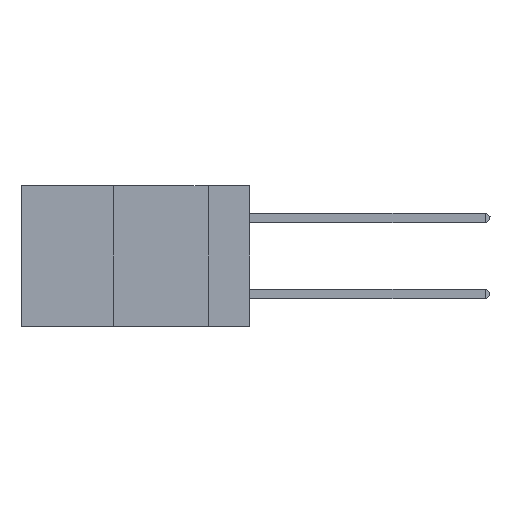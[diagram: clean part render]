
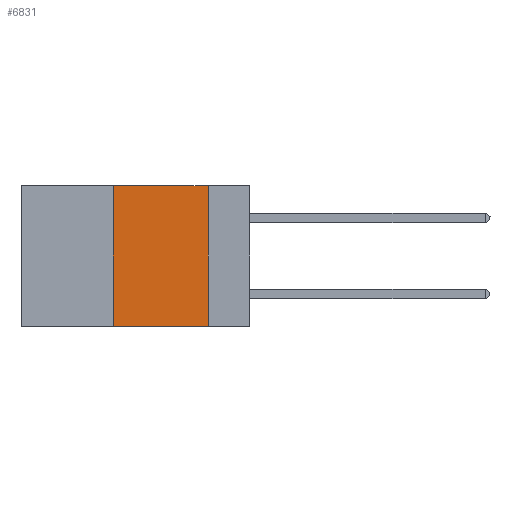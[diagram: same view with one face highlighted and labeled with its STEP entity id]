
A CAD part, left-side view. The second image highlights one B-rep face of the part: STEP entity #6831.
In plain terms, the highlighted planar face has unit normal (-1, 0, 0).
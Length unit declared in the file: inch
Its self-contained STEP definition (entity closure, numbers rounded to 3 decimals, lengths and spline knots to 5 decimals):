
#839 = CARTESIAN_POINT ( 'NONE',  ( 0., 0.6, 0. ) ) ;
#938 = CARTESIAN_POINT ( 'NONE',  ( 0., 0.11, 0. ) ) ;
#1014 = DIRECTION ( 'NONE',  ( 0., 0., -1. ) ) ;
#1046 = DIRECTION ( 'NONE',  ( 0., -1., 0. ) ) ;
#2424 = PLANE ( 'NONE',  #3870 ) ;
#2739 = CARTESIAN_POINT ( 'NONE',  ( 0., 0.11, 0. ) ) ;
#2751 = CARTESIAN_POINT ( 'NONE',  ( 0., 0.36, 0. ) ) ;
#3157 = VECTOR ( 'NONE', #1014, 39.37008 ) ;
#3190 = ORIENTED_EDGE ( 'NONE', *, *, #15618, .F. ) ;
#3303 = VERTEX_POINT ( 'NONE', #2739 ) ;
#3870 = AXIS2_PLACEMENT_3D ( 'NONE', #839, #15048, #6884 ) ;
#4284 = CARTESIAN_POINT ( 'NONE',  ( 0., 0.11, -0.37 ) ) ;
#4734 = EDGE_LOOP ( 'NONE', ( #8311, #4740, #3190, #5533 ) ) ;
#4740 = ORIENTED_EDGE ( 'NONE', *, *, #17905, .F. ) ;
#5424 = LINE ( 'NONE', #5764, #15921 ) ;
#5504 = EDGE_CURVE ( 'NONE', #3303, #11034, #7060, .T. ) ;
#5533 = ORIENTED_EDGE ( 'NONE', *, *, #14988, .T. ) ;
#5764 = CARTESIAN_POINT ( 'NONE',  ( 0., 0.6, -0.37 ) ) ;
#6831 = ADVANCED_FACE ( 'NONE', ( #10636 ), #2424, .F. ) ;
#6884 = DIRECTION ( 'NONE',  ( 0., 0., -1. ) ) ;
#7060 = LINE ( 'NONE', #938, #3157 ) ;
#7329 = LINE ( 'NONE', #12550, #10985 ) ;
#7344 = CARTESIAN_POINT ( 'NONE',  ( 0., 0.36, 0. ) ) ;
#7450 = VERTEX_POINT ( 'NONE', #13889 ) ;
#7642 = LINE ( 'NONE', #2751, #10868 ) ;
#8311 = ORIENTED_EDGE ( 'NONE', *, *, #5504, .F. ) ;
#9996 = DIRECTION ( 'NONE',  ( 0., -1., 0. ) ) ;
#10636 = FACE_OUTER_BOUND ( 'NONE', #4734, .T. ) ;
#10868 = VECTOR ( 'NONE', #16653, 39.37008 ) ;
#10985 = VECTOR ( 'NONE', #1046, 39.37008 ) ;
#11034 = VERTEX_POINT ( 'NONE', #4284 ) ;
#12550 = CARTESIAN_POINT ( 'NONE',  ( 0., 0.6, 0. ) ) ;
#13889 = CARTESIAN_POINT ( 'NONE',  ( 0., 0.36, -0.37 ) ) ;
#14988 = EDGE_CURVE ( 'NONE', #7450, #11034, #5424, .T. ) ;
#15048 = DIRECTION ( 'NONE',  ( 1., 0., 0. ) ) ;
#15618 = EDGE_CURVE ( 'NONE', #7450, #16768, #7642, .T. ) ;
#15921 = VECTOR ( 'NONE', #9996, 39.37008 ) ;
#16653 = DIRECTION ( 'NONE',  ( 0., 0., 1. ) ) ;
#16768 = VERTEX_POINT ( 'NONE', #7344 ) ;
#17905 = EDGE_CURVE ( 'NONE', #16768, #3303, #7329, .T. ) ;
